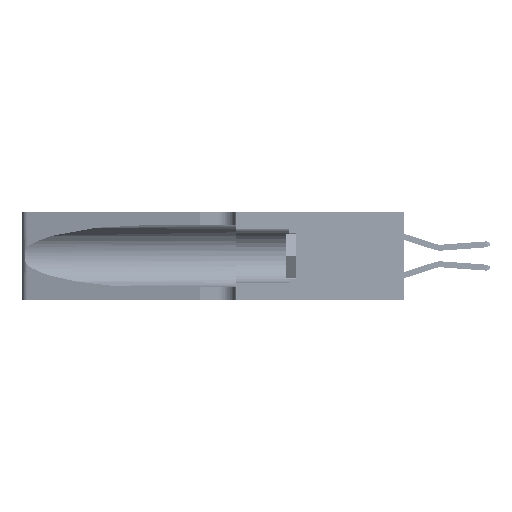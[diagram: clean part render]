
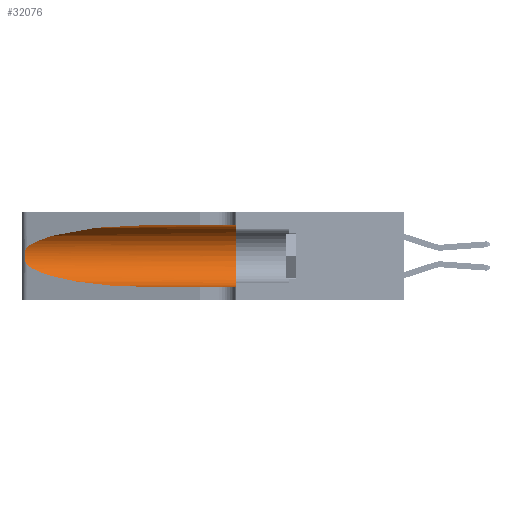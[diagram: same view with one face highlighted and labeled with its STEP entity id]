
A CAD part, left-side view. The second image highlights one B-rep face of the part: STEP entity #32076.
In plain terms, the highlighted cylindrical face has radius 3.308 mm (diameter 6.617 mm), a partial arc.
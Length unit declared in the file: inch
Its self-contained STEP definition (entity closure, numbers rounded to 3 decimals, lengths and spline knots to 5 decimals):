
#455 = CARTESIAN_POINT ( 'NONE',  ( 0.25487, 1.22718, 0.14631 ) ) ;
#525 = VECTOR ( 'NONE', #21318, 39.37008 ) ;
#2352 = CARTESIAN_POINT ( 'NONE',  ( 0.2373, 1.15595, 0.08982 ) ) ;
#4142 = CARTESIAN_POINT ( 'NONE',  ( 0.26017, 1.23833, 0.17102 ) ) ;
#4538 = EDGE_CURVE ( 'NONE', #9702, #37583, #27553, .T. ) ;
#4831 = CARTESIAN_POINT ( 'NONE',  ( 0.25555, 1.22994, 0.2215 ) ) ;
#5553 = EDGE_CURVE ( 'NONE', #21863, #9702, #44007, .T. ) ;
#5876 = EDGE_CURVE ( 'NONE', #21863, #31597, #11225, .T. ) ;
#7640 = DIRECTION ( 'NONE',  ( 0., -1., 0. ) ) ;
#8192 = CARTESIAN_POINT ( 'NONE',  ( 0.25487, 1.22718, 0.22369 ) ) ;
#8354 = CARTESIAN_POINT ( 'NONE',  ( 0.26075, 1.23896, 0.178 ) ) ;
#8890 = CIRCLE ( 'NONE', #43068, 0.13025 ) ;
#9702 = VERTEX_POINT ( 'NONE', #22303 ) ;
#9797 = CARTESIAN_POINT ( 'NONE',  ( 0.1305, 0.35, 0.185 ) ) ;
#11179 = CARTESIAN_POINT ( 'NONE',  ( 0.1305, 0.72297, 0.05475 ) ) ;
#11225 = LINE ( 'NONE', #45492, #525 ) ;
#11689 = LINE ( 'NONE', #28754, #23073 ) ;
#12577 = CARTESIAN_POINT ( 'NONE',  ( 0.25856, 1.23593, 0.16098 ) ) ;
#13161 = ORIENTED_EDGE ( 'NONE', *, *, #5553, .T. ) ;
#15258 = ORIENTED_EDGE ( 'NONE', *, *, #19288, .T. ) ;
#15866 =( BOUNDED_CURVE ( )  B_SPLINE_CURVE ( 3, ( #30412, #2352, #34295, #42913 ),
 .UNSPECIFIED., .F., .F. ) 
 B_SPLINE_CURVE_WITH_KNOTS ( ( 4, 4 ),
 ( 3.44316, 4.71239 ),
 .UNSPECIFIED. ) 
 CURVE ( )  GEOMETRIC_REPRESENTATION_ITEM ( )  RATIONAL_B_SPLINE_CURVE ( ( 1., 0.87, 0.87, 1. ) ) 
 REPRESENTATION_ITEM ( '' )  );
#17550 = DIRECTION ( 'NONE',  ( 0., 0., 1. ) ) ;
#18507 = CARTESIAN_POINT ( 'NONE',  ( 0.1305, 0.72297, 0.31525 ) ) ;
#18664 = CARTESIAN_POINT ( 'NONE',  ( 0.1305, 0.72297, 0.31525 ) ) ;
#19288 = EDGE_CURVE ( 'NONE', #36185, #40118, #11689, .T. ) ;
#20540 = CARTESIAN_POINT ( 'NONE',  ( 0.25639, 1.23184, 0.21858 ) ) ;
#21318 = DIRECTION ( 'NONE',  ( 0., -1., 0. ) ) ;
#21863 = VERTEX_POINT ( 'NONE', #18664 ) ;
#22002 = ORIENTED_EDGE ( 'NONE', *, *, #49124, .F. ) ;
#22235 = CARTESIAN_POINT ( 'NONE',  ( 0.18966, 0.96281, 0.31525 ) ) ;
#22303 = CARTESIAN_POINT ( 'NONE',  ( 0.25487, 1.22718, 0.22369 ) ) ;
#22854 = EDGE_LOOP ( 'NONE', ( #13161, #37101, #47319, #15258, #22002, #44705 ) ) ;
#23073 = VECTOR ( 'NONE', #40202, 39.37008 ) ;
#24649 = CARTESIAN_POINT ( 'NONE',  ( 0.25789, 1.23486, 0.15765 ) ) ;
#26855 = CARTESIAN_POINT ( 'NONE',  ( 0.25487, 1.22718, 0.22369 ) ) ;
#27553 = B_SPLINE_CURVE_WITH_KNOTS ( 'NONE', 3,
 ( #8192, #4831, #20540, #36767, #40987, #49139, #32727, #8354, #4142, #12577, #24649, #28324, #28833, #455 ),
 .UNSPECIFIED., .F., .F.,
 ( 4, 2, 2, 2, 2, 2, 4 ),
 ( 0., 0.00027, 0.00053, 0.00107, 0.0016, 0.00187, 0.00214 ),
 .UNSPECIFIED. ) ;
#27731 = AXIS2_PLACEMENT_3D ( 'NONE', #51779, #7640, #27792 ) ;
#27792 = DIRECTION ( 'NONE',  ( 0., 0., -1. ) ) ;
#28324 = CARTESIAN_POINT ( 'NONE',  ( 0.25639, 1.23186, 0.15144 ) ) ;
#28754 = CARTESIAN_POINT ( 'NONE',  ( 0.1305, 1.61858, 0.05475 ) ) ;
#28833 = CARTESIAN_POINT ( 'NONE',  ( 0.25555, 1.22993, 0.14849 ) ) ;
#30412 = CARTESIAN_POINT ( 'NONE',  ( 0.25487, 1.22718, 0.14631 ) ) ;
#31597 = VERTEX_POINT ( 'NONE', #45458 ) ;
#32076 = ADVANCED_FACE ( 'NONE', ( #42510 ), #48206, .F. ) ;
#32727 = CARTESIAN_POINT ( 'NONE',  ( 0.26075, 1.23896, 0.19203 ) ) ;
#34295 = CARTESIAN_POINT ( 'NONE',  ( 0.18966, 0.96281, 0.05475 ) ) ;
#35600 = CARTESIAN_POINT ( 'NONE',  ( 0.1305, 0.35, 0.05475 ) ) ;
#36185 = VERTEX_POINT ( 'NONE', #11179 ) ;
#36767 = CARTESIAN_POINT ( 'NONE',  ( 0.25787, 1.23484, 0.2124 ) ) ;
#37101 = ORIENTED_EDGE ( 'NONE', *, *, #4538, .T. ) ;
#37583 = VERTEX_POINT ( 'NONE', #48478 ) ;
#38611 = CARTESIAN_POINT ( 'NONE',  ( 0.2373, 1.15595, 0.28018 ) ) ;
#40118 = VERTEX_POINT ( 'NONE', #35600 ) ;
#40202 = DIRECTION ( 'NONE',  ( 0., -1., 0. ) ) ;
#40987 = CARTESIAN_POINT ( 'NONE',  ( 0.25854, 1.2359, 0.20912 ) ) ;
#42510 = FACE_OUTER_BOUND ( 'NONE', #22854, .T. ) ;
#42913 = CARTESIAN_POINT ( 'NONE',  ( 0.1305, 0.72297, 0.05475 ) ) ;
#43068 = AXIS2_PLACEMENT_3D ( 'NONE', #9797, #45446, #17550 ) ;
#44007 =( BOUNDED_CURVE ( )  B_SPLINE_CURVE ( 3, ( #18507, #22235, #38611, #26855 ),
 .UNSPECIFIED., .F., .F. ) 
 B_SPLINE_CURVE_WITH_KNOTS ( ( 4, 4 ),
 ( 1.5708, 2.84003 ),
 .UNSPECIFIED. ) 
 CURVE ( )  GEOMETRIC_REPRESENTATION_ITEM ( )  RATIONAL_B_SPLINE_CURVE ( ( 1., 0.87, 0.87, 1. ) ) 
 REPRESENTATION_ITEM ( '' )  );
#44705 = ORIENTED_EDGE ( 'NONE', *, *, #5876, .F. ) ;
#45446 = DIRECTION ( 'NONE',  ( 0., 1., 0. ) ) ;
#45458 = CARTESIAN_POINT ( 'NONE',  ( 0.1305, 0.35, 0.31525 ) ) ;
#45492 = CARTESIAN_POINT ( 'NONE',  ( 0.1305, 1.61858, 0.31525 ) ) ;
#47319 = ORIENTED_EDGE ( 'NONE', *, *, #48603, .T. ) ;
#48206 = CYLINDRICAL_SURFACE ( 'NONE', #27731, 0.13025 ) ;
#48478 = CARTESIAN_POINT ( 'NONE',  ( 0.25487, 1.22718, 0.14631 ) ) ;
#48603 = EDGE_CURVE ( 'NONE', #37583, #36185, #15866, .T. ) ;
#49124 = EDGE_CURVE ( 'NONE', #31597, #40118, #8890, .T. ) ;
#49139 = CARTESIAN_POINT ( 'NONE',  ( 0.26018, 1.23835, 0.19895 ) ) ;
#51779 = CARTESIAN_POINT ( 'NONE',  ( 0.1305, 1.61858, 0.185 ) ) ;
